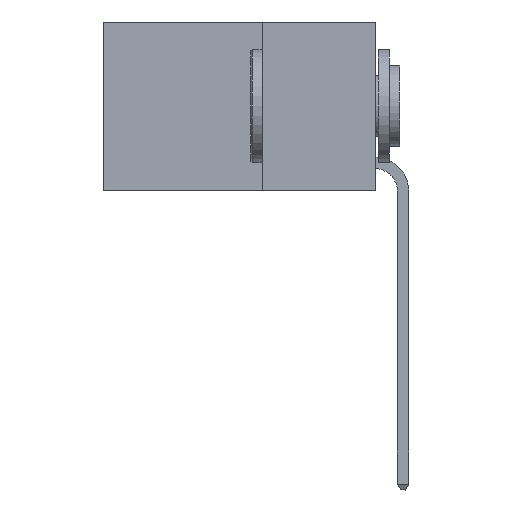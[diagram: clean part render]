
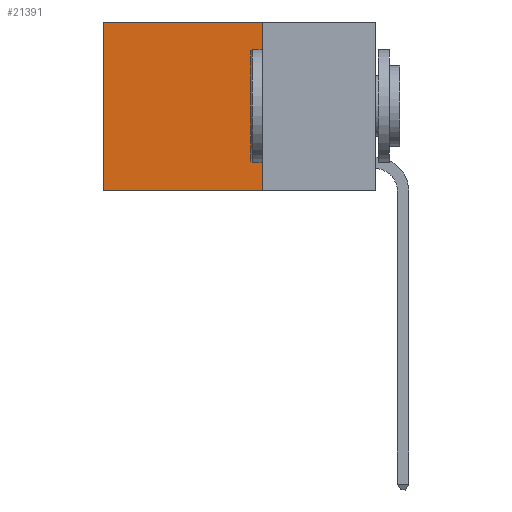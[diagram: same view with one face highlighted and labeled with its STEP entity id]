
A CAD part, left-side view. The second image highlights one B-rep face of the part: STEP entity #21391.
In plain terms, the highlighted planar face has unit normal (-1, 0, 0).
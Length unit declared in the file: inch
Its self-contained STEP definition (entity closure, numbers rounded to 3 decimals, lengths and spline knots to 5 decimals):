
#83 = CARTESIAN_POINT ( 'NONE',  ( 0.2625, 0.25, -0.37 ) ) ;
#182 = CARTESIAN_POINT ( 'NONE',  ( 0.2625, 0.25, 0. ) ) ;
#186 = CARTESIAN_POINT ( 'NONE',  ( 0.2625, 0.25, 0. ) ) ;
#200 = AXIS2_PLACEMENT_3D ( 'NONE', #20755, #9154, #22687 ) ;
#2508 = VERTEX_POINT ( 'NONE', #21503 ) ;
#5163 = PLANE ( 'NONE',  #200 ) ;
#5876 = ORIENTED_EDGE ( 'NONE', *, *, #22270, .F. ) ;
#7513 = CARTESIAN_POINT ( 'NONE',  ( 0.2625, 0.6, 0. ) ) ;
#7919 = VERTEX_POINT ( 'NONE', #23628 ) ;
#8491 = ORIENTED_EDGE ( 'NONE', *, *, #20486, .T. ) ;
#9154 = DIRECTION ( 'NONE',  ( 1., 0., 0. ) ) ;
#9162 = VECTOR ( 'NONE', #15934, 39.37008 ) ;
#9182 = ORIENTED_EDGE ( 'NONE', *, *, #21496, .T. ) ;
#9937 = VECTOR ( 'NONE', #14065, 39.37008 ) ;
#10248 = DIRECTION ( 'NONE',  ( 0., 1., 0. ) ) ;
#10434 = EDGE_CURVE ( 'NONE', #2508, #7919, #19494, .T. ) ;
#10842 = ORIENTED_EDGE ( 'NONE', *, *, #10434, .F. ) ;
#11095 = EDGE_LOOP ( 'NONE', ( #9182, #10842, #5876, #8491 ) ) ;
#11796 = CARTESIAN_POINT ( 'NONE',  ( 0.2625, 0.25, 0. ) ) ;
#14065 = DIRECTION ( 'NONE',  ( 0., 0., -1. ) ) ;
#14175 = VERTEX_POINT ( 'NONE', #11796 ) ;
#14276 = CARTESIAN_POINT ( 'NONE',  ( 0.2625, 0.6, 0. ) ) ;
#15934 = DIRECTION ( 'NONE',  ( 0., 1., 0. ) ) ;
#16453 = VECTOR ( 'NONE', #10248, 39.37008 ) ;
#16680 = LINE ( 'NONE', #7513, #21175 ) ;
#17042 = LINE ( 'NONE', #182, #16453 ) ;
#19494 = LINE ( 'NONE', #83, #9162 ) ;
#20486 = EDGE_CURVE ( 'NONE', #14175, #24970, #17042, .T. ) ;
#20755 = CARTESIAN_POINT ( 'NONE',  ( 0.2625, 0.25, 0. ) ) ;
#21175 = VECTOR ( 'NONE', #23021, 39.37008 ) ;
#21391 = ADVANCED_FACE ( 'NONE', ( #24205 ), #5163, .F. ) ;
#21496 = EDGE_CURVE ( 'NONE', #24970, #7919, #16680, .T. ) ;
#21503 = CARTESIAN_POINT ( 'NONE',  ( 0.2625, 0.25, -0.37 ) ) ;
#22270 = EDGE_CURVE ( 'NONE', #14175, #2508, #24741, .T. ) ;
#22687 = DIRECTION ( 'NONE',  ( 0., 0., -1. ) ) ;
#23021 = DIRECTION ( 'NONE',  ( 0., 0., -1. ) ) ;
#23628 = CARTESIAN_POINT ( 'NONE',  ( 0.2625, 0.6, -0.37 ) ) ;
#24205 = FACE_OUTER_BOUND ( 'NONE', #11095, .T. ) ;
#24741 = LINE ( 'NONE', #186, #9937 ) ;
#24970 = VERTEX_POINT ( 'NONE', #14276 ) ;
